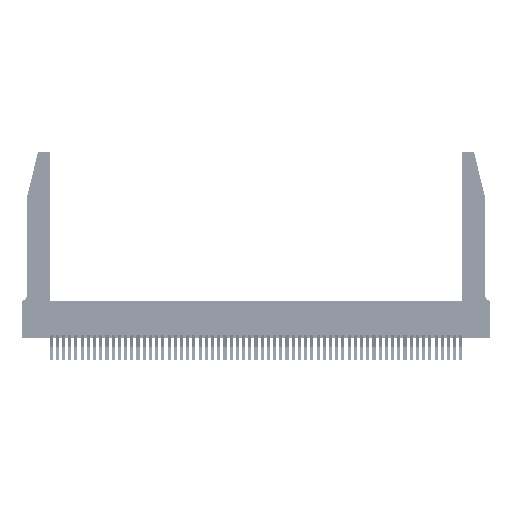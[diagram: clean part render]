
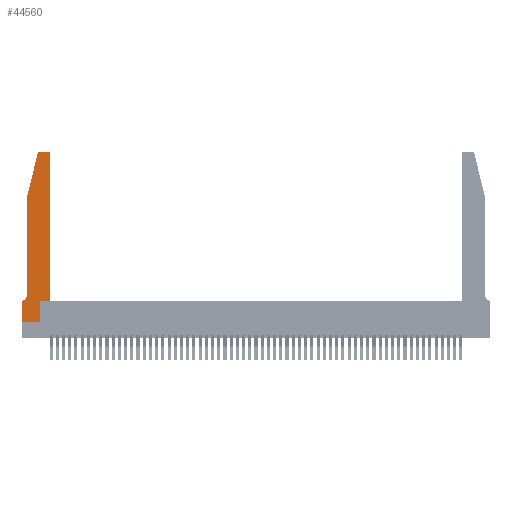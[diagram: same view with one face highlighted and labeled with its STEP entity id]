
A CAD part, top view. The second image highlights one B-rep face of the part: STEP entity #44560.
In plain terms, the highlighted planar face has unit normal (0, 0, 1).
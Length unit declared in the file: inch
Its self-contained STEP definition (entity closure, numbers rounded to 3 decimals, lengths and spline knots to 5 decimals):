
#139 = PLANE ( 'NONE',  #30157 ) ;
#643 = ORIENTED_EDGE ( 'NONE', *, *, #11723, .T. ) ;
#677 = CARTESIAN_POINT ( 'NONE',  ( 0., 0., 0.37 ) ) ;
#934 = VERTEX_POINT ( 'NONE', #23005 ) ;
#1905 = CARTESIAN_POINT ( 'NONE',  ( 0.0055, 0.42, 0.37 ) ) ;
#2705 = EDGE_CURVE ( 'NONE', #13671, #14881, #43809, .T. ) ;
#2863 = VECTOR ( 'NONE', #18781, 39.37008 ) ;
#3050 = CARTESIAN_POINT ( 'NONE',  ( 0.0055, 0.35, 0.37 ) ) ;
#5374 = DIRECTION ( 'NONE',  ( -1., 0., 0. ) ) ;
#5431 = DIRECTION ( 'NONE',  ( 1., 0., 0. ) ) ;
#5479 = VERTEX_POINT ( 'NONE', #53083 ) ;
#6142 = DIRECTION ( 'NONE',  ( 0., 0., 1. ) ) ;
#6373 = CARTESIAN_POINT ( 'NONE',  ( 0.0755, 2., 0.37 ) ) ;
#6594 = EDGE_CURVE ( 'NONE', #934, #5479, #8139, .T. ) ;
#8117 = AXIS2_PLACEMENT_3D ( 'NONE', #26836, #6142, #35556 ) ;
#8139 = LINE ( 'NONE', #18598, #2863 ) ;
#8643 = DIRECTION ( 'NONE',  ( -1., 0., 0. ) ) ;
#9206 = CARTESIAN_POINT ( 'NONE',  ( 0.0755, 0.35, 0.37 ) ) ;
#10259 = CIRCLE ( 'NONE', #14754, 0.07 ) ;
#10452 = ORIENTED_EDGE ( 'NONE', *, *, #29384, .T. ) ;
#10912 = DIRECTION ( 'NONE',  ( 0., 1., 0. ) ) ;
#10973 = EDGE_CURVE ( 'NONE', #20801, #19399, #21414, .T. ) ;
#11489 = ORIENTED_EDGE ( 'NONE', *, *, #2705, .T. ) ;
#11723 = EDGE_CURVE ( 'NONE', #12980, #20801, #43116, .T. ) ;
#11885 = EDGE_CURVE ( 'NONE', #46632, #934, #20306, .T. ) ;
#12330 = FACE_OUTER_BOUND ( 'NONE', #33483, .T. ) ;
#12980 = VERTEX_POINT ( 'NONE', #53544 ) ;
#13580 = VECTOR ( 'NONE', #16073, 39.37008 ) ;
#13671 = VERTEX_POINT ( 'NONE', #32747 ) ;
#13856 = VERTEX_POINT ( 'NONE', #43269 ) ;
#13888 = DIRECTION ( 'NONE',  ( 0., 0., -1. ) ) ;
#14550 = LINE ( 'NONE', #43719, #16469 ) ;
#14684 = LINE ( 'NONE', #677, #46567 ) ;
#14754 = AXIS2_PLACEMENT_3D ( 'NONE', #1905, #13888, #5374 ) ;
#14881 = VERTEX_POINT ( 'NONE', #40784 ) ;
#16073 = DIRECTION ( 'NONE',  ( -1., 0., 0. ) ) ;
#16204 = ORIENTED_EDGE ( 'NONE', *, *, #33638, .T. ) ;
#16469 = VECTOR ( 'NONE', #10912, 39.37008 ) ;
#16796 = CARTESIAN_POINT ( 'NONE',  ( 0.2605, 2.75, 0.37 ) ) ;
#16945 = ORIENTED_EDGE ( 'NONE', *, *, #6594, .T. ) ;
#17100 = DIRECTION ( 'NONE',  ( 1., 0., 0. ) ) ;
#18598 = CARTESIAN_POINT ( 'NONE',  ( 0.4505, 0.35, 0.37 ) ) ;
#18781 = DIRECTION ( 'NONE',  ( 1., 0., 0. ) ) ;
#19170 = ORIENTED_EDGE ( 'NONE', *, *, #40653, .T. ) ;
#19399 = VERTEX_POINT ( 'NONE', #22313 ) ;
#19984 = ORIENTED_EDGE ( 'NONE', *, *, #10973, .T. ) ;
#20165 = CIRCLE ( 'NONE', #8117, 0.03 ) ;
#20306 = LINE ( 'NONE', #21477, #34603 ) ;
#20801 = VERTEX_POINT ( 'NONE', #48360 ) ;
#21414 = LINE ( 'NONE', #16796, #13580 ) ;
#21477 = CARTESIAN_POINT ( 'NONE',  ( 0.2865, 0.35, 0.37 ) ) ;
#22313 = CARTESIAN_POINT ( 'NONE',  ( 0.284, 2.75, 0.37 ) ) ;
#22329 = CARTESIAN_POINT ( 'NONE',  ( 0.0755, 2., 0.37 ) ) ;
#22386 = CARTESIAN_POINT ( 'NONE',  ( 0., 0., 0.37 ) ) ;
#22764 = CARTESIAN_POINT ( 'NONE',  ( 0., 0.35, 0.37 ) ) ;
#23005 = CARTESIAN_POINT ( 'NONE',  ( 0.2865, 0.35, 0.37 ) ) ;
#24190 = EDGE_CURVE ( 'NONE', #14881, #37294, #31290, .T. ) ;
#25177 = VECTOR ( 'NONE', #43481, 39.37008 ) ;
#25476 = CARTESIAN_POINT ( 'NONE',  ( 0.4205, 2.72, 0.37 ) ) ;
#26670 = DIRECTION ( 'NONE',  ( -0.239, -0.971, 0. ) ) ;
#26836 = CARTESIAN_POINT ( 'NONE',  ( 0.284, 2.72, 0.37 ) ) ;
#29384 = EDGE_CURVE ( 'NONE', #13856, #46632, #14684, .T. ) ;
#29479 = DIRECTION ( 'NONE',  ( 0., 0., 1. ) ) ;
#30157 = AXIS2_PLACEMENT_3D ( 'NONE', #42153, #33612, #50352 ) ;
#31042 = DIRECTION ( 'NONE',  ( 0., -1., 0. ) ) ;
#31290 = LINE ( 'NONE', #6373, #46255 ) ;
#31721 = ORIENTED_EDGE ( 'NONE', *, *, #46546, .T. ) ;
#32736 = VECTOR ( 'NONE', #26670, 39.37008 ) ;
#32747 = CARTESIAN_POINT ( 'NONE',  ( 0.25487, 2.72718, 0.37 ) ) ;
#33483 = EDGE_LOOP ( 'NONE', ( #19984, #16204, #11489, #51750, #52347, #31721, #44052, #10452, #37571, #16945, #19170, #643 ) ) ;
#33612 = DIRECTION ( 'NONE',  ( 0., 0., 1. ) ) ;
#33638 = EDGE_CURVE ( 'NONE', #19399, #13671, #20165, .T. ) ;
#33751 = CARTESIAN_POINT ( 'NONE',  ( 0.0755, 0.42, 0.37 ) ) ;
#34603 = VECTOR ( 'NONE', #42726, 39.37008 ) ;
#35556 = DIRECTION ( 'NONE',  ( 1., 0., 0. ) ) ;
#36200 = EDGE_CURVE ( 'NONE', #44280, #13856, #45984, .T. ) ;
#37294 = VERTEX_POINT ( 'NONE', #33751 ) ;
#37571 = ORIENTED_EDGE ( 'NONE', *, *, #11885, .T. ) ;
#39129 = VERTEX_POINT ( 'NONE', #3050 ) ;
#40653 = EDGE_CURVE ( 'NONE', #5479, #12980, #14550, .T. ) ;
#40784 = CARTESIAN_POINT ( 'NONE',  ( 0.0755, 2., 0.37 ) ) ;
#42153 = CARTESIAN_POINT ( 'NONE',  ( 0., 0.35, 0.37 ) ) ;
#42550 = CARTESIAN_POINT ( 'NONE',  ( 0.2865, 0., 0.37 ) ) ;
#42726 = DIRECTION ( 'NONE',  ( 0., 1., 0. ) ) ;
#43116 = CIRCLE ( 'NONE', #50412, 0.03 ) ;
#43269 = CARTESIAN_POINT ( 'NONE',  ( 0., 0., 0.37 ) ) ;
#43481 = DIRECTION ( 'NONE',  ( 0., -1., 0. ) ) ;
#43696 = EDGE_CURVE ( 'NONE', #37294, #39129, #10259, .T. ) ;
#43719 = CARTESIAN_POINT ( 'NONE',  ( 0.4505, 0.35, 0.37 ) ) ;
#43809 = LINE ( 'NONE', #22329, #32736 ) ;
#44052 = ORIENTED_EDGE ( 'NONE', *, *, #36200, .T. ) ;
#44280 = VERTEX_POINT ( 'NONE', #22764 ) ;
#44560 = ADVANCED_FACE ( 'NONE', ( #12330 ), #139, .T. ) ;
#44719 = LINE ( 'NONE', #9206, #51245 ) ;
#45984 = LINE ( 'NONE', #22386, #25177 ) ;
#46255 = VECTOR ( 'NONE', #31042, 39.37008 ) ;
#46546 = EDGE_CURVE ( 'NONE', #39129, #44280, #44719, .T. ) ;
#46567 = VECTOR ( 'NONE', #5431, 39.37008 ) ;
#46632 = VERTEX_POINT ( 'NONE', #42550 ) ;
#48360 = CARTESIAN_POINT ( 'NONE',  ( 0.4205, 2.75, 0.37 ) ) ;
#50352 = DIRECTION ( 'NONE',  ( 1., 0., 0. ) ) ;
#50412 = AXIS2_PLACEMENT_3D ( 'NONE', #25476, #29479, #17100 ) ;
#51245 = VECTOR ( 'NONE', #8643, 39.37008 ) ;
#51750 = ORIENTED_EDGE ( 'NONE', *, *, #24190, .T. ) ;
#52347 = ORIENTED_EDGE ( 'NONE', *, *, #43696, .T. ) ;
#53083 = CARTESIAN_POINT ( 'NONE',  ( 0.4505, 0.35, 0.37 ) ) ;
#53544 = CARTESIAN_POINT ( 'NONE',  ( 0.4505, 2.72, 0.37 ) ) ;
